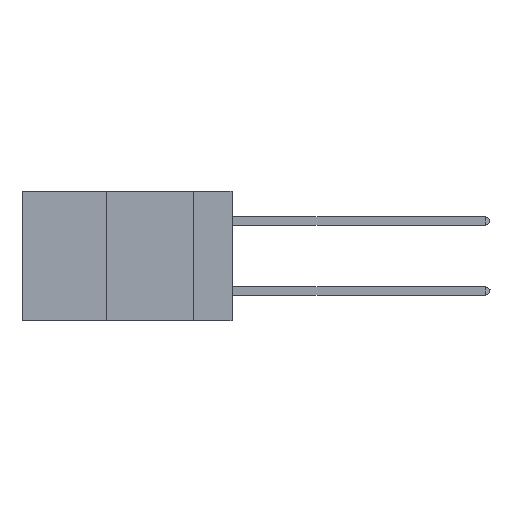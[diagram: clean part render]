
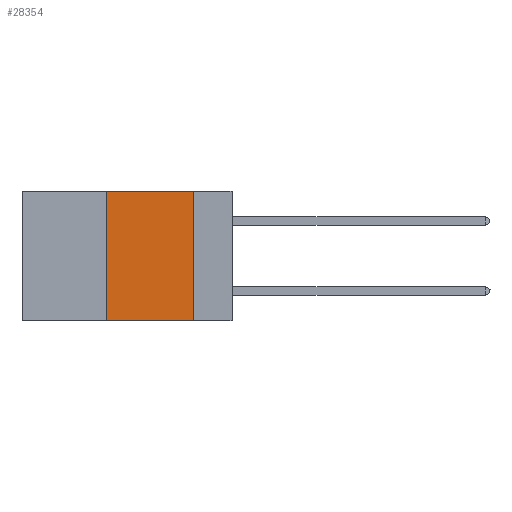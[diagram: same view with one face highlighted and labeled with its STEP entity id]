
A CAD part, left-side view. The second image highlights one B-rep face of the part: STEP entity #28354.
In plain terms, the highlighted planar face has unit normal (-1, 0, 0).
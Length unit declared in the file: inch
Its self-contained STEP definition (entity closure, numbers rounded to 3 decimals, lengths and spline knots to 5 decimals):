
#1203 = EDGE_CURVE ( 'NONE', #13685, #21603, #3886, .T. ) ;
#3740 = CARTESIAN_POINT ( 'NONE',  ( 0., 0.6, 0. ) ) ;
#3886 = LINE ( 'NONE', #10535, #34494 ) ;
#4448 = CARTESIAN_POINT ( 'NONE',  ( 0., 0.11, 0. ) ) ;
#10080 = ORIENTED_EDGE ( 'NONE', *, *, #1203, .F. ) ;
#10264 = DIRECTION ( 'NONE',  ( 1., 0., 0. ) ) ;
#10332 = LINE ( 'NONE', #17881, #35356 ) ;
#10535 = CARTESIAN_POINT ( 'NONE',  ( 0., 0.11, 0. ) ) ;
#10671 = DIRECTION ( 'NONE',  ( 0., 0., -1. ) ) ;
#10955 = CARTESIAN_POINT ( 'NONE',  ( 0., 0.11, -0.37 ) ) ;
#11916 = ORIENTED_EDGE ( 'NONE', *, *, #11964, .F. ) ;
#11964 = EDGE_CURVE ( 'NONE', #34205, #13685, #10332, .T. ) ;
#12014 = AXIS2_PLACEMENT_3D ( 'NONE', #3740, #10264, #13552 ) ;
#13552 = DIRECTION ( 'NONE',  ( 0., 0., -1. ) ) ;
#13685 = VERTEX_POINT ( 'NONE', #4448 ) ;
#13687 = LINE ( 'NONE', #40783, #36661 ) ;
#14405 = DIRECTION ( 'NONE',  ( 0., 0., 1. ) ) ;
#16660 = CARTESIAN_POINT ( 'NONE',  ( 0., 0.6, -0.37 ) ) ;
#16890 = CARTESIAN_POINT ( 'NONE',  ( 0., 0.36, 0. ) ) ;
#17881 = CARTESIAN_POINT ( 'NONE',  ( 0., 0.6, 0. ) ) ;
#17984 = CARTESIAN_POINT ( 'NONE',  ( 0., 0.36, -0.37 ) ) ;
#19128 = EDGE_CURVE ( 'NONE', #26182, #34205, #13687, .T. ) ;
#19953 = DIRECTION ( 'NONE',  ( 0., -1., 0. ) ) ;
#21565 = DIRECTION ( 'NONE',  ( 0., -1., 0. ) ) ;
#21603 = VERTEX_POINT ( 'NONE', #10955 ) ;
#22629 = ORIENTED_EDGE ( 'NONE', *, *, #19128, .F. ) ;
#23176 = EDGE_LOOP ( 'NONE', ( #10080, #11916, #22629, #39505 ) ) ;
#26182 = VERTEX_POINT ( 'NONE', #17984 ) ;
#27969 = VECTOR ( 'NONE', #19953, 39.37008 ) ;
#28354 = ADVANCED_FACE ( 'NONE', ( #33079 ), #29690, .F. ) ;
#29028 = EDGE_CURVE ( 'NONE', #26182, #21603, #36657, .T. ) ;
#29690 = PLANE ( 'NONE',  #12014 ) ;
#33079 = FACE_OUTER_BOUND ( 'NONE', #23176, .T. ) ;
#34205 = VERTEX_POINT ( 'NONE', #16890 ) ;
#34494 = VECTOR ( 'NONE', #10671, 39.37008 ) ;
#35356 = VECTOR ( 'NONE', #21565, 39.37008 ) ;
#36657 = LINE ( 'NONE', #16660, #27969 ) ;
#36661 = VECTOR ( 'NONE', #14405, 39.37008 ) ;
#39505 = ORIENTED_EDGE ( 'NONE', *, *, #29028, .T. ) ;
#40783 = CARTESIAN_POINT ( 'NONE',  ( 0., 0.36, 0. ) ) ;
